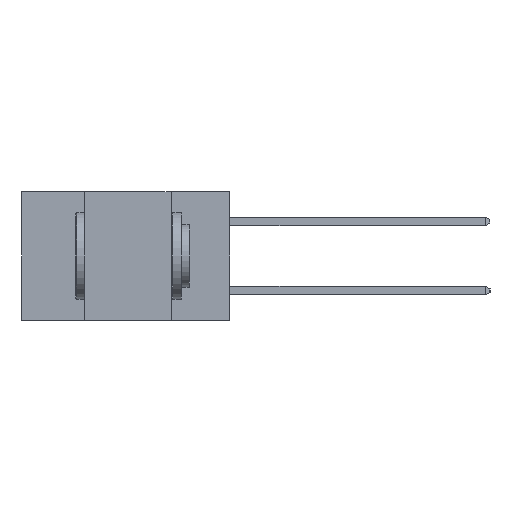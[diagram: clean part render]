
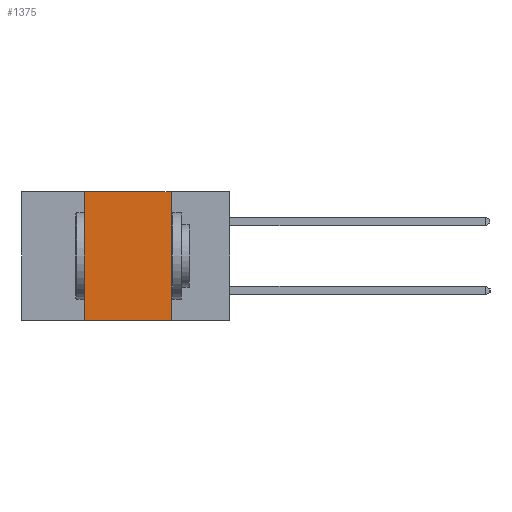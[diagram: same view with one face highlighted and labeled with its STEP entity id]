
A CAD part, left-side view. The second image highlights one B-rep face of the part: STEP entity #1375.
In plain terms, the highlighted planar face has unit normal (-1, 0, 0).
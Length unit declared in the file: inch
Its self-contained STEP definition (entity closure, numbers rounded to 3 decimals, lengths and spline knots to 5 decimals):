
#13 = VERTEX_POINT ( 'NONE', #11999 ) ;
#759 = CARTESIAN_POINT ( 'NONE',  ( 0., 0.17, -0.37 ) ) ;
#1104 = LINE ( 'NONE', #759, #6445 ) ;
#1274 = VECTOR ( 'NONE', #7361, 39.37008 ) ;
#1375 = ADVANCED_FACE ( 'NONE', ( #11873 ), #11427, .F. ) ;
#1448 = LINE ( 'NONE', #1585, #4065 ) ;
#1585 = CARTESIAN_POINT ( 'NONE',  ( 0., 0.42, -0.37 ) ) ;
#1756 = VERTEX_POINT ( 'NONE', #3730 ) ;
#1982 = LINE ( 'NONE', #2071, #1274 ) ;
#2071 = CARTESIAN_POINT ( 'NONE',  ( 0., 0.6, 0. ) ) ;
#2723 = DIRECTION ( 'NONE',  ( 0., 0., 1. ) ) ;
#3039 = CARTESIAN_POINT ( 'NONE',  ( 0., 0.17, -0.37 ) ) ;
#3730 = CARTESIAN_POINT ( 'NONE',  ( 0., 0.42, -0.37 ) ) ;
#4065 = VECTOR ( 'NONE', #2723, 39.37008 ) ;
#4311 = ORIENTED_EDGE ( 'NONE', *, *, #11109, .F. ) ;
#4487 = ORIENTED_EDGE ( 'NONE', *, *, #10957, .F. ) ;
#4835 = VERTEX_POINT ( 'NONE', #3039 ) ;
#5970 = CARTESIAN_POINT ( 'NONE',  ( 0., 0.6, -0.37 ) ) ;
#6117 = VECTOR ( 'NONE', #12886, 39.37008 ) ;
#6445 = VECTOR ( 'NONE', #9197, 39.37008 ) ;
#6641 = DIRECTION ( 'NONE',  ( 0., 0., -1. ) ) ;
#7201 = DIRECTION ( 'NONE',  ( 1., 0., 0. ) ) ;
#7361 = DIRECTION ( 'NONE',  ( 0., -1., 0. ) ) ;
#7933 = EDGE_LOOP ( 'NONE', ( #4487, #4311, #11107, #10164 ) ) ;
#8786 = CARTESIAN_POINT ( 'NONE',  ( 0., 0.6, 0. ) ) ;
#9197 = DIRECTION ( 'NONE',  ( 0., 0., -1. ) ) ;
#9740 = CARTESIAN_POINT ( 'NONE',  ( 0., 0.42, 0. ) ) ;
#10164 = ORIENTED_EDGE ( 'NONE', *, *, #11464, .T. ) ;
#10957 = EDGE_CURVE ( 'NONE', #13, #4835, #1104, .T. ) ;
#11107 = ORIENTED_EDGE ( 'NONE', *, *, #11373, .F. ) ;
#11109 = EDGE_CURVE ( 'NONE', #11240, #13, #1982, .T. ) ;
#11153 = LINE ( 'NONE', #5970, #6117 ) ;
#11240 = VERTEX_POINT ( 'NONE', #9740 ) ;
#11323 = AXIS2_PLACEMENT_3D ( 'NONE', #8786, #7201, #6641 ) ;
#11373 = EDGE_CURVE ( 'NONE', #1756, #11240, #1448, .T. ) ;
#11427 = PLANE ( 'NONE',  #11323 ) ;
#11464 = EDGE_CURVE ( 'NONE', #1756, #4835, #11153, .T. ) ;
#11873 = FACE_OUTER_BOUND ( 'NONE', #7933, .T. ) ;
#11999 = CARTESIAN_POINT ( 'NONE',  ( 0., 0.17, 0. ) ) ;
#12886 = DIRECTION ( 'NONE',  ( 0., -1., 0. ) ) ;
